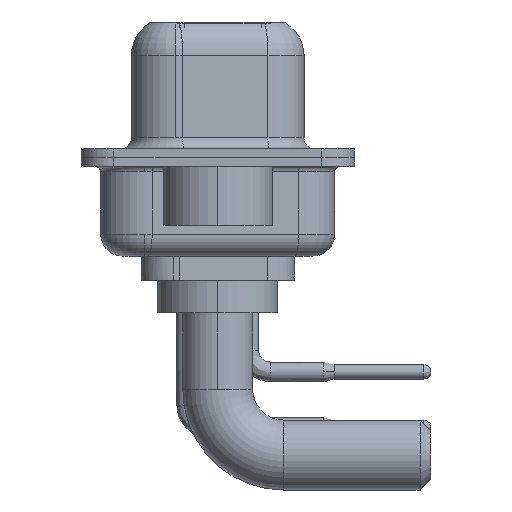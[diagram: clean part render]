
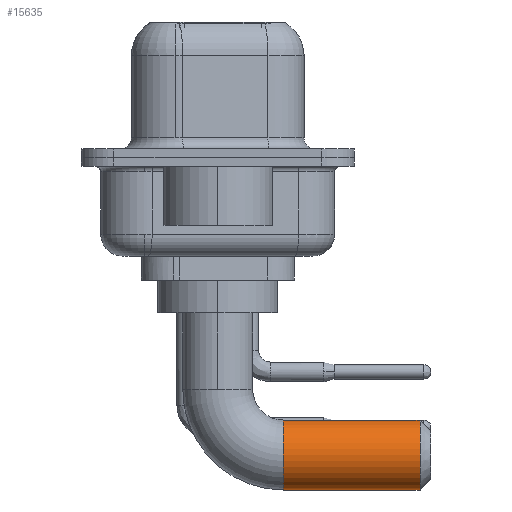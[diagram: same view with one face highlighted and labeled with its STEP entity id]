
A CAD part, left-side view. The second image highlights one B-rep face of the part: STEP entity #15635.
In plain terms, the highlighted cylindrical face has radius 1.6 mm (diameter 3.2 mm), a partial arc.
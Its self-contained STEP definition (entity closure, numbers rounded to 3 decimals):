
#118 = CARTESIAN_POINT ( 'NONE',  ( 0., -3., -6.5 ) ) ;
#732 = VECTOR ( 'NONE', #5047, 1000. ) ;
#1004 = VERTEX_POINT ( 'NONE', #20088 ) ;
#1054 = CARTESIAN_POINT ( 'NONE',  ( 0., -3., -4.9 ) ) ;
#1798 = CYLINDRICAL_SURFACE ( 'NONE', #23215, 1.6 ) ;
#3881 = LINE ( 'NONE', #16411, #9492 ) ;
#4687 = LINE ( 'NONE', #1054, #732 ) ;
#5047 = DIRECTION ( 'NONE',  ( 0., -1., 0. ) ) ;
#5187 = CIRCLE ( 'NONE', #23483, 1.6 ) ;
#5248 = VERTEX_POINT ( 'NONE', #5802 ) ;
#5802 = CARTESIAN_POINT ( 'NONE',  ( 0., -3., -8.1 ) ) ;
#6196 = DIRECTION ( 'NONE',  ( -1., 0., 0. ) ) ;
#7473 = DIRECTION ( 'NONE',  ( 0., -1., 0. ) ) ;
#7614 = ORIENTED_EDGE ( 'NONE', *, *, #12560, .F. ) ;
#8513 = ORIENTED_EDGE ( 'NONE', *, *, #11518, .T. ) ;
#8529 = CARTESIAN_POINT ( 'NONE',  ( 0., -9.25, -4.9 ) ) ;
#8996 = EDGE_CURVE ( 'NONE', #5248, #18338, #3881, .T. ) ;
#9492 = VECTOR ( 'NONE', #23800, 1000. ) ;
#11518 = EDGE_CURVE ( 'NONE', #1004, #5248, #5187, .T. ) ;
#12560 = EDGE_CURVE ( 'NONE', #1004, #13985, #4687, .T. ) ;
#13411 = DIRECTION ( 'NONE',  ( 0., -1., 0. ) ) ;
#13985 = VERTEX_POINT ( 'NONE', #8529 ) ;
#14454 = ORIENTED_EDGE ( 'NONE', *, *, #8996, .T. ) ;
#14834 = DIRECTION ( 'NONE',  ( 0., 0., -1. ) ) ;
#15635 = ADVANCED_FACE ( 'NONE', ( #18334 ), #1798, .T. ) ;
#16411 = CARTESIAN_POINT ( 'NONE',  ( 0., -3., -8.1 ) ) ;
#16688 = AXIS2_PLACEMENT_3D ( 'NONE', #17378, #21947, #19553 ) ;
#17283 = CARTESIAN_POINT ( 'NONE',  ( 0., -9.25, -8.1 ) ) ;
#17344 = EDGE_LOOP ( 'NONE', ( #7614, #8513, #14454, #17472 ) ) ;
#17378 = CARTESIAN_POINT ( 'NONE',  ( 0., -9.25, -6.5 ) ) ;
#17472 = ORIENTED_EDGE ( 'NONE', *, *, #17543, .T. ) ;
#17543 = EDGE_CURVE ( 'NONE', #18338, #13985, #20949, .T. ) ;
#18334 = FACE_OUTER_BOUND ( 'NONE', #17344, .T. ) ;
#18338 = VERTEX_POINT ( 'NONE', #17283 ) ;
#19553 = DIRECTION ( 'NONE',  ( 0., 0., -1. ) ) ;
#20088 = CARTESIAN_POINT ( 'NONE',  ( 0., -3., -4.9 ) ) ;
#20949 = CIRCLE ( 'NONE', #16688, 1.6 ) ;
#21947 = DIRECTION ( 'NONE',  ( 0., 1., 0. ) ) ;
#22951 = CARTESIAN_POINT ( 'NONE',  ( 0., -3., -6.5 ) ) ;
#23215 = AXIS2_PLACEMENT_3D ( 'NONE', #118, #7473, #14834 ) ;
#23483 = AXIS2_PLACEMENT_3D ( 'NONE', #22951, #13411, #6196 ) ;
#23800 = DIRECTION ( 'NONE',  ( 0., -1., 0. ) ) ;
